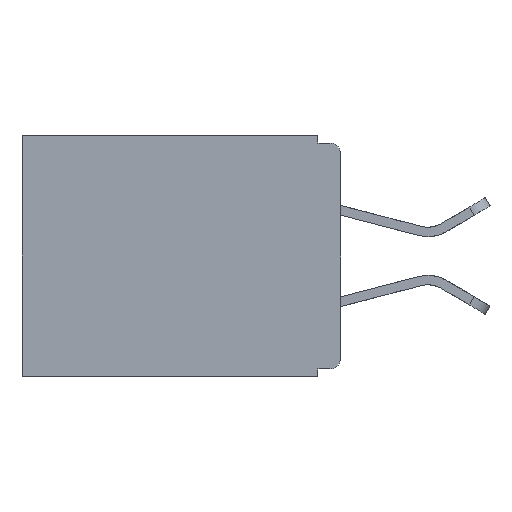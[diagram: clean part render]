
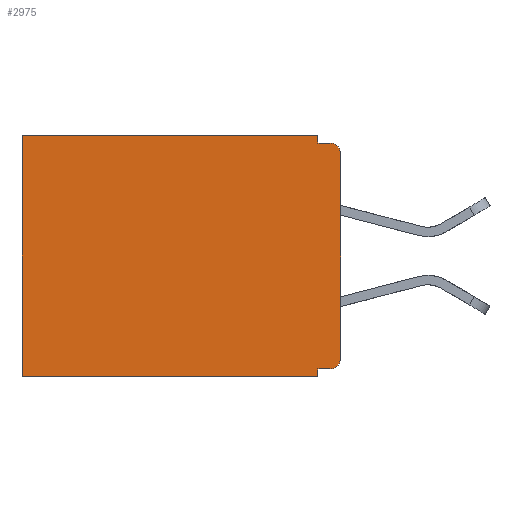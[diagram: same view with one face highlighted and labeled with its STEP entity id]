
A CAD part, left-side view. The second image highlights one B-rep face of the part: STEP entity #2975.
In plain terms, the highlighted planar face has unit normal (-1, 0, 0).
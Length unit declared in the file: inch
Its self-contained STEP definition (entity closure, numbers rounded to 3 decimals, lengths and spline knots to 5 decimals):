
#347 = VECTOR ( 'NONE', #21888, 39.37008 ) ;
#599 = ORIENTED_EDGE ( 'NONE', *, *, #10068, .F. ) ;
#662 = ORIENTED_EDGE ( 'NONE', *, *, #15929, .T. ) ;
#798 = FACE_OUTER_BOUND ( 'NONE', #23255, .T. ) ;
#1752 = DIRECTION ( 'NONE',  ( 0., 0., -1. ) ) ;
#1758 = DIRECTION ( 'NONE',  ( -1., 0., 0. ) ) ;
#1814 = CARTESIAN_POINT ( 'NONE',  ( 0.3, 0.015, -0.025 ) ) ;
#2150 = AXIS2_PLACEMENT_3D ( 'NONE', #1814, #1758, #1752 ) ;
#2164 = VERTEX_POINT ( 'NONE', #9156 ) ;
#2169 = VECTOR ( 'NONE', #13440, 39.37008 ) ;
#2975 = ADVANCED_FACE ( 'NONE', ( #798 ), #22899, .F. ) ;
#3181 = VECTOR ( 'NONE', #23004, 39.37008 ) ;
#3627 = ORIENTED_EDGE ( 'NONE', *, *, #18731, .F. ) ;
#4923 = CIRCLE ( 'NONE', #11922, 0.015 ) ;
#4975 = VECTOR ( 'NONE', #13070, 39.37008 ) ;
#5521 = VECTOR ( 'NONE', #9865, 39.37008 ) ;
#5916 = DIRECTION ( 'NONE',  ( 0., 0., -1. ) ) ;
#5943 = CARTESIAN_POINT ( 'NONE',  ( 0.3, 0.437, -0.33 ) ) ;
#6251 = CARTESIAN_POINT ( 'NONE',  ( 0.3, 0.031, 0. ) ) ;
#7368 = VECTOR ( 'NONE', #5916, 39.37008 ) ;
#7565 = ORIENTED_EDGE ( 'NONE', *, *, #9150, .T. ) ;
#7688 = LINE ( 'NONE', #21725, #17784 ) ;
#8110 = EDGE_CURVE ( 'NONE', #17305, #10434, #18753, .T. ) ;
#8499 = AXIS2_PLACEMENT_3D ( 'NONE', #14346, #10831, #10715 ) ;
#8622 = LINE ( 'NONE', #6251, #7368 ) ;
#9150 = EDGE_CURVE ( 'NONE', #9341, #10434, #21726, .T. ) ;
#9156 = CARTESIAN_POINT ( 'NONE',  ( 0.3, 0.031, -0.01 ) ) ;
#9341 = VERTEX_POINT ( 'NONE', #19388 ) ;
#9379 = VERTEX_POINT ( 'NONE', #19181 ) ;
#9732 = CARTESIAN_POINT ( 'NONE',  ( 0.3, 0.031, -0.33 ) ) ;
#9790 = DIRECTION ( 'NONE',  ( -1., 0., 0. ) ) ;
#9865 = DIRECTION ( 'NONE',  ( 0., 1., 0. ) ) ;
#9887 = CARTESIAN_POINT ( 'NONE',  ( 0.3, 0., -0.32 ) ) ;
#10068 = EDGE_CURVE ( 'NONE', #23980, #14180, #14964, .T. ) ;
#10209 = CARTESIAN_POINT ( 'NONE',  ( 0.3, 0.015, -0.01 ) ) ;
#10434 = VERTEX_POINT ( 'NONE', #5943 ) ;
#10715 = DIRECTION ( 'NONE',  ( 0., 0., -1. ) ) ;
#10831 = DIRECTION ( 'NONE',  ( 1., 0., 0. ) ) ;
#10946 = LINE ( 'NONE', #11067, #4975 ) ;
#11067 = CARTESIAN_POINT ( 'NONE',  ( 0.3, 0., -0.01 ) ) ;
#11899 = EDGE_CURVE ( 'NONE', #14658, #20116, #7688, .T. ) ;
#11922 = AXIS2_PLACEMENT_3D ( 'NONE', #21942, #9790, #23928 ) ;
#12061 = ORIENTED_EDGE ( 'NONE', *, *, #15440, .T. ) ;
#13070 = DIRECTION ( 'NONE',  ( 0., -1., 0. ) ) ;
#13183 = ORIENTED_EDGE ( 'NONE', *, *, #8110, .F. ) ;
#13236 = CARTESIAN_POINT ( 'NONE',  ( 0.3, 0., 0. ) ) ;
#13440 = DIRECTION ( 'NONE',  ( 0., 1., 0. ) ) ;
#14180 = VERTEX_POINT ( 'NONE', #23939 ) ;
#14346 = CARTESIAN_POINT ( 'NONE',  ( 0.3, 0., -0.33 ) ) ;
#14562 = CARTESIAN_POINT ( 'NONE',  ( 0.3, 0.031, -0.33 ) ) ;
#14658 = VERTEX_POINT ( 'NONE', #15346 ) ;
#14964 = LINE ( 'NONE', #9887, #5521 ) ;
#15346 = CARTESIAN_POINT ( 'NONE',  ( 0.3, 0., -0.025 ) ) ;
#15440 = EDGE_CURVE ( 'NONE', #14658, #23069, #19081, .T. ) ;
#15781 = ORIENTED_EDGE ( 'NONE', *, *, #19602, .T. ) ;
#15929 = EDGE_CURVE ( 'NONE', #9379, #9341, #23131, .T. ) ;
#16157 = EDGE_CURVE ( 'NONE', #9379, #2164, #8622, .T. ) ;
#16297 = VECTOR ( 'NONE', #21956, 39.37008 ) ;
#16629 = LINE ( 'NONE', #9732, #347 ) ;
#17305 = VERTEX_POINT ( 'NONE', #14562 ) ;
#17784 = VECTOR ( 'NONE', #21696, 39.37008 ) ;
#18731 = EDGE_CURVE ( 'NONE', #2164, #23069, #10946, .T. ) ;
#18753 = LINE ( 'NONE', #21607, #3181 ) ;
#18939 = EDGE_CURVE ( 'NONE', #14180, #17305, #16629, .T. ) ;
#19081 = CIRCLE ( 'NONE', #2150, 0.015 ) ;
#19121 = ORIENTED_EDGE ( 'NONE', *, *, #11899, .F. ) ;
#19181 = CARTESIAN_POINT ( 'NONE',  ( 0.3, 0.031, 0. ) ) ;
#19388 = CARTESIAN_POINT ( 'NONE',  ( 0.3, 0.437, 0. ) ) ;
#19602 = EDGE_CURVE ( 'NONE', #23980, #20116, #4923, .T. ) ;
#19695 = CARTESIAN_POINT ( 'NONE',  ( 0.3, 0.015, -0.32 ) ) ;
#20116 = VERTEX_POINT ( 'NONE', #25421 ) ;
#21143 = ORIENTED_EDGE ( 'NONE', *, *, #18939, .F. ) ;
#21607 = CARTESIAN_POINT ( 'NONE',  ( 0.3, 0., -0.33 ) ) ;
#21696 = DIRECTION ( 'NONE',  ( 0., 0., -1. ) ) ;
#21725 = CARTESIAN_POINT ( 'NONE',  ( 0.3, 0., -0.33 ) ) ;
#21726 = LINE ( 'NONE', #21753, #16297 ) ;
#21753 = CARTESIAN_POINT ( 'NONE',  ( 0.3, 0.437, -0.33 ) ) ;
#21888 = DIRECTION ( 'NONE',  ( 0., 0., -1. ) ) ;
#21942 = CARTESIAN_POINT ( 'NONE',  ( 0.3, 0.015, -0.305 ) ) ;
#21956 = DIRECTION ( 'NONE',  ( 0., 0., -1. ) ) ;
#22899 = PLANE ( 'NONE',  #8499 ) ;
#23004 = DIRECTION ( 'NONE',  ( 0., 1., 0. ) ) ;
#23069 = VERTEX_POINT ( 'NONE', #10209 ) ;
#23131 = LINE ( 'NONE', #13236, #2169 ) ;
#23255 = EDGE_LOOP ( 'NONE', ( #19121, #12061, #3627, #24009, #662, #7565, #13183, #21143, #599, #15781 ) ) ;
#23928 = DIRECTION ( 'NONE',  ( 0., 0., -1. ) ) ;
#23939 = CARTESIAN_POINT ( 'NONE',  ( 0.3, 0.031, -0.32 ) ) ;
#23980 = VERTEX_POINT ( 'NONE', #19695 ) ;
#24009 = ORIENTED_EDGE ( 'NONE', *, *, #16157, .F. ) ;
#25421 = CARTESIAN_POINT ( 'NONE',  ( 0.3, 0., -0.305 ) ) ;
